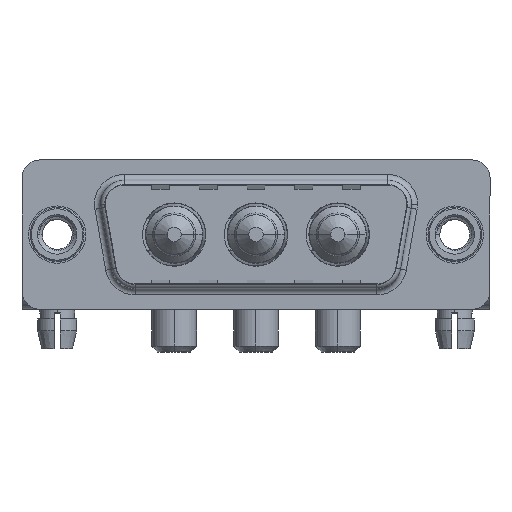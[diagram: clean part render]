
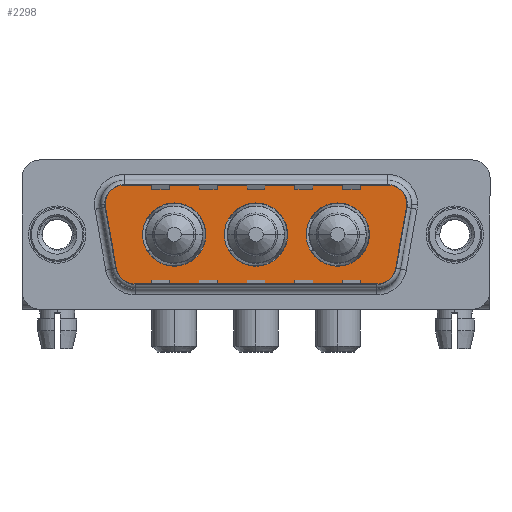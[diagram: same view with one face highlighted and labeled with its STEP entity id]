
A CAD part, top view. The second image highlights one B-rep face of the part: STEP entity #2298.
In plain terms, the highlighted planar face has unit normal (0, 0, 1).
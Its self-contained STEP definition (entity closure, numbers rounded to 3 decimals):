
#85 = EDGE_CURVE ( 'NONE', #1647, #13062, #11402, .T. ) ;
#248 = CARTESIAN_POINT ( 'NONE',  ( 3.441, 2.553, 0. ) ) ;
#330 = CARTESIAN_POINT ( 'NONE',  ( 23.5, 0., 0. ) ) ;
#551 = CARTESIAN_POINT ( 'NONE',  ( 14., 0., 0. ) ) ;
#553 = FACE_BOUND ( 'NONE', #9354, .T. ) ;
#649 = DIRECTION ( 'NONE',  ( 1., 0., 0. ) ) ;
#719 = CARTESIAN_POINT ( 'NONE',  ( 27.889, 2.9, 0. ) ) ;
#754 = CIRCLE ( 'NONE', #8156, 2. ) ;
#897 = DIRECTION ( 'NONE',  ( -1., 0., 0. ) ) ;
#1140 = ORIENTED_EDGE ( 'NONE', *, *, #5395, .F. ) ;
#1190 = DIRECTION ( 'NONE',  ( 0., 0., 1. ) ) ;
#1317 = LINE ( 'NONE', #13097, #3312 ) ;
#1377 = EDGE_LOOP ( 'NONE', ( #9822, #15262 ) ) ;
#1526 = AXIS2_PLACEMENT_3D ( 'NONE', #330, #10484, #12036 ) ;
#1529 = CARTESIAN_POINT ( 'NONE',  ( 6.434, -4.9, 0. ) ) ;
#1541 = ORIENTED_EDGE ( 'NONE', *, *, #85, .T. ) ;
#1647 = VERTEX_POINT ( 'NONE', #1529 ) ;
#1655 = EDGE_CURVE ( 'NONE', #15222, #5848, #13222, .T. ) ;
#2011 = FACE_BOUND ( 'NONE', #1377, .T. ) ;
#2298 = ADVANCED_FACE ( 'NONE', ( #2011, #13804, #553, #4751 ), #4417, .T. ) ;
#2595 = VECTOR ( 'NONE', #649, 1000. ) ;
#2626 = CARTESIAN_POINT ( 'NONE',  ( 6.434, -2.9, 0. ) ) ;
#2717 = CARTESIAN_POINT ( 'NONE',  ( 20.85, 0., 0. ) ) ;
#3208 = DIRECTION ( 'NONE',  ( 0., 0., 1. ) ) ;
#3312 = VECTOR ( 'NONE', #10338, 1000. ) ;
#3637 = DIRECTION ( 'NONE',  ( 0., 0., 1. ) ) ;
#3680 = CIRCLE ( 'NONE', #6682, 2.65 ) ;
#3943 = EDGE_CURVE ( 'NONE', #7126, #4092, #3680, .T. ) ;
#4092 = VERTEX_POINT ( 'NONE', #13174 ) ;
#4102 = DIRECTION ( 'NONE',  ( 1., 0., 0. ) ) ;
#4417 = PLANE ( 'NONE',  #12522 ) ;
#4632 = AXIS2_PLACEMENT_3D ( 'NONE', #2626, #16696, #8859 ) ;
#4711 = CARTESIAN_POINT ( 'NONE',  ( 12.45, 0., 0. ) ) ;
#4751 = FACE_OUTER_BOUND ( 'NONE', #7978, .T. ) ;
#5070 = VERTEX_POINT ( 'NONE', #7724 ) ;
#5221 = CARTESIAN_POINT ( 'NONE',  ( 26.866, -2.9, 0. ) ) ;
#5395 = EDGE_CURVE ( 'NONE', #5848, #15222, #7834, .T. ) ;
#5448 = DIRECTION ( 'NONE',  ( 0., 0., 1. ) ) ;
#5462 = CARTESIAN_POINT ( 'NONE',  ( 5.411, 4.9, 0. ) ) ;
#5520 = LINE ( 'NONE', #12322, #6504 ) ;
#5537 = DIRECTION ( 'NONE',  ( -1., 0., 0. ) ) ;
#5566 = ORIENTED_EDGE ( 'NONE', *, *, #7641, .T. ) ;
#5747 = ORIENTED_EDGE ( 'NONE', *, *, #8691, .T. ) ;
#5848 = VERTEX_POINT ( 'NONE', #2717 ) ;
#5960 = CARTESIAN_POINT ( 'NONE',  ( 5.411, 2.9, 0. ) ) ;
#6045 = CARTESIAN_POINT ( 'NONE',  ( 26.866, -2.9, 0. ) ) ;
#6125 = VERTEX_POINT ( 'NONE', #5462 ) ;
#6504 = VECTOR ( 'NONE', #9408, 1000. ) ;
#6535 = CIRCLE ( 'NONE', #12072, 2.65 ) ;
#6682 = AXIS2_PLACEMENT_3D ( 'NONE', #8958, #12751, #7573 ) ;
#6695 = ORIENTED_EDGE ( 'NONE', *, *, #8476, .T. ) ;
#6750 = CARTESIAN_POINT ( 'NONE',  ( 5.411, 4.9, 0. ) ) ;
#6762 = ORIENTED_EDGE ( 'NONE', *, *, #14622, .F. ) ;
#6806 = AXIS2_PLACEMENT_3D ( 'NONE', #5960, #16573, #8556 ) ;
#6894 = CARTESIAN_POINT ( 'NONE',  ( 9.8, 0., 0. ) ) ;
#7002 = EDGE_CURVE ( 'NONE', #5070, #7176, #8483, .T. ) ;
#7118 = EDGE_CURVE ( 'NONE', #7789, #12269, #6535, .T. ) ;
#7126 = VERTEX_POINT ( 'NONE', #551 ) ;
#7176 = VERTEX_POINT ( 'NONE', #11054 ) ;
#7546 = DIRECTION ( 'NONE',  ( 1., 0., 0. ) ) ;
#7573 = DIRECTION ( 'NONE',  ( 1., 0., 0. ) ) ;
#7630 = CARTESIAN_POINT ( 'NONE',  ( 16.65, 0., 0. ) ) ;
#7641 = EDGE_CURVE ( 'NONE', #15536, #5070, #5520, .T. ) ;
#7724 = CARTESIAN_POINT ( 'NONE',  ( 29.859, 2.553, 0. ) ) ;
#7789 = VERTEX_POINT ( 'NONE', #8698 ) ;
#7834 = CIRCLE ( 'NONE', #1526, 2.65 ) ;
#7974 = AXIS2_PLACEMENT_3D ( 'NONE', #10734, #16001, #4102 ) ;
#7978 = EDGE_LOOP ( 'NONE', ( #12523, #5566, #13165, #9229, #15023, #5747, #13580, #6695, #1541 ) ) ;
#8028 = DIRECTION ( 'NONE',  ( 1., 0., 0. ) ) ;
#8115 = CARTESIAN_POINT ( 'NONE',  ( 27.889, 2.9, 0. ) ) ;
#8156 = AXIS2_PLACEMENT_3D ( 'NONE', #719, #3637, #897 ) ;
#8325 = VERTEX_POINT ( 'NONE', #11355 ) ;
#8449 = CARTESIAN_POINT ( 'NONE',  ( 27.889, 4.9, 0. ) ) ;
#8476 = EDGE_CURVE ( 'NONE', #8325, #1647, #12070, .T. ) ;
#8483 = CIRCLE ( 'NONE', #9580, 2. ) ;
#8551 = DIRECTION ( 'NONE',  ( 1., 0., 0. ) ) ;
#8556 = DIRECTION ( 'NONE',  ( 1., 0., 0. ) ) ;
#8691 = EDGE_CURVE ( 'NONE', #6125, #15606, #12885, .T. ) ;
#8698 = CARTESIAN_POINT ( 'NONE',  ( 7.15, 0., 0. ) ) ;
#8718 = CIRCLE ( 'NONE', #10634, 2.65 ) ;
#8859 = DIRECTION ( 'NONE',  ( -1., 0., 0. ) ) ;
#8958 = CARTESIAN_POINT ( 'NONE',  ( 16.65, 0., 0. ) ) ;
#9229 = ORIENTED_EDGE ( 'NONE', *, *, #11980, .T. ) ;
#9330 = DIRECTION ( 'NONE',  ( 0., 0., 1. ) ) ;
#9354 = EDGE_LOOP ( 'NONE', ( #6762, #16325 ) ) ;
#9408 = DIRECTION ( 'NONE',  ( 0.174, 0.985, 0. ) ) ;
#9580 = AXIS2_PLACEMENT_3D ( 'NONE', #8115, #5448, #5537 ) ;
#9809 = EDGE_CURVE ( 'NONE', #16228, #6125, #16245, .T. ) ;
#9822 = ORIENTED_EDGE ( 'NONE', *, *, #12375, .F. ) ;
#10338 = DIRECTION ( 'NONE',  ( 0.174, -0.985, 0. ) ) ;
#10484 = DIRECTION ( 'NONE',  ( 0., 0., 1. ) ) ;
#10497 = AXIS2_PLACEMENT_3D ( 'NONE', #6894, #9330, #8028 ) ;
#10634 = AXIS2_PLACEMENT_3D ( 'NONE', #7630, #1190, #7546 ) ;
#10734 = CARTESIAN_POINT ( 'NONE',  ( 23.5, 0., 0. ) ) ;
#11054 = CARTESIAN_POINT ( 'NONE',  ( 29.889, 2.9, 0. ) ) ;
#11069 = DIRECTION ( 'NONE',  ( -1., 0., 0. ) ) ;
#11203 = CIRCLE ( 'NONE', #14490, 2. ) ;
#11355 = CARTESIAN_POINT ( 'NONE',  ( 4.464, -3.247, 0. ) ) ;
#11402 = LINE ( 'NONE', #13989, #2595 ) ;
#11954 = EDGE_LOOP ( 'NONE', ( #17018, #1140 ) ) ;
#11980 = EDGE_CURVE ( 'NONE', #7176, #16228, #754, .T. ) ;
#12036 = DIRECTION ( 'NONE',  ( 1., 0., 0. ) ) ;
#12070 = CIRCLE ( 'NONE', #4632, 2. ) ;
#12072 = AXIS2_PLACEMENT_3D ( 'NONE', #12427, #3208, #16308 ) ;
#12155 = CIRCLE ( 'NONE', #10497, 2.65 ) ;
#12269 = VERTEX_POINT ( 'NONE', #4711 ) ;
#12322 = CARTESIAN_POINT ( 'NONE',  ( 29.859, 2.553, 0. ) ) ;
#12375 = EDGE_CURVE ( 'NONE', #4092, #7126, #8718, .T. ) ;
#12427 = CARTESIAN_POINT ( 'NONE',  ( 9.8, 0., 0. ) ) ;
#12522 = AXIS2_PLACEMENT_3D ( 'NONE', #6045, #15011, #8551 ) ;
#12523 = ORIENTED_EDGE ( 'NONE', *, *, #12600, .T. ) ;
#12600 = EDGE_CURVE ( 'NONE', #13062, #15536, #11203, .T. ) ;
#12751 = DIRECTION ( 'NONE',  ( 0., 0., 1. ) ) ;
#12885 = CIRCLE ( 'NONE', #6806, 2. ) ;
#12986 = CARTESIAN_POINT ( 'NONE',  ( 28.836, -3.247, 0. ) ) ;
#13062 = VERTEX_POINT ( 'NONE', #15719 ) ;
#13097 = CARTESIAN_POINT ( 'NONE',  ( 3.441, 2.553, 0. ) ) ;
#13165 = ORIENTED_EDGE ( 'NONE', *, *, #7002, .T. ) ;
#13174 = CARTESIAN_POINT ( 'NONE',  ( 19.3, 0., 0. ) ) ;
#13222 = CIRCLE ( 'NONE', #7974, 2.65 ) ;
#13521 = EDGE_CURVE ( 'NONE', #15606, #8325, #1317, .T. ) ;
#13580 = ORIENTED_EDGE ( 'NONE', *, *, #13521, .T. ) ;
#13804 = FACE_BOUND ( 'NONE', #11954, .T. ) ;
#13989 = CARTESIAN_POINT ( 'NONE',  ( 6.434, -4.9, 0. ) ) ;
#14434 = DIRECTION ( 'NONE',  ( 1., 0., 0. ) ) ;
#14490 = AXIS2_PLACEMENT_3D ( 'NONE', #5221, #15739, #14434 ) ;
#14622 = EDGE_CURVE ( 'NONE', #12269, #7789, #12155, .T. ) ;
#15011 = DIRECTION ( 'NONE',  ( 0., 0., 1. ) ) ;
#15023 = ORIENTED_EDGE ( 'NONE', *, *, #9809, .T. ) ;
#15222 = VERTEX_POINT ( 'NONE', #15856 ) ;
#15262 = ORIENTED_EDGE ( 'NONE', *, *, #3943, .F. ) ;
#15536 = VERTEX_POINT ( 'NONE', #12986 ) ;
#15606 = VERTEX_POINT ( 'NONE', #248 ) ;
#15719 = CARTESIAN_POINT ( 'NONE',  ( 26.866, -4.9, 0. ) ) ;
#15739 = DIRECTION ( 'NONE',  ( 0., 0., 1. ) ) ;
#15856 = CARTESIAN_POINT ( 'NONE',  ( 26.15, 0., 0. ) ) ;
#15947 = VECTOR ( 'NONE', #11069, 1000. ) ;
#16001 = DIRECTION ( 'NONE',  ( 0., 0., 1. ) ) ;
#16228 = VERTEX_POINT ( 'NONE', #8449 ) ;
#16245 = LINE ( 'NONE', #6750, #15947 ) ;
#16308 = DIRECTION ( 'NONE',  ( 1., 0., 0. ) ) ;
#16325 = ORIENTED_EDGE ( 'NONE', *, *, #7118, .F. ) ;
#16573 = DIRECTION ( 'NONE',  ( 0., 0., 1. ) ) ;
#16696 = DIRECTION ( 'NONE',  ( 0., 0., 1. ) ) ;
#17018 = ORIENTED_EDGE ( 'NONE', *, *, #1655, .F. ) ;
